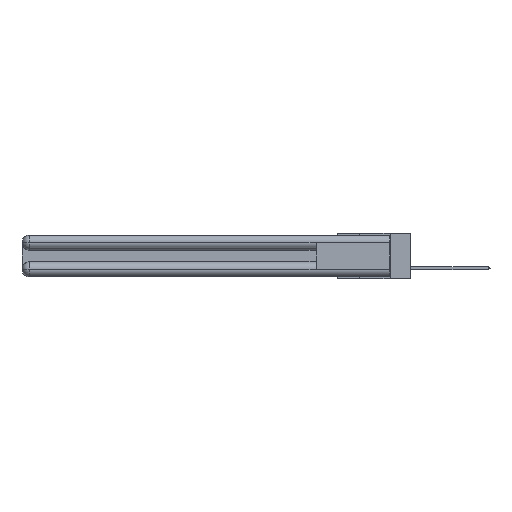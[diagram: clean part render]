
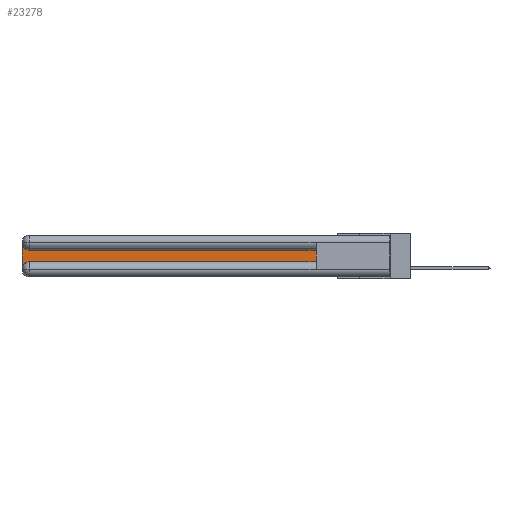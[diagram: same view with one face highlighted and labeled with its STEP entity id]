
A CAD part, left-side view. The second image highlights one B-rep face of the part: STEP entity #23278.
In plain terms, the highlighted planar face has unit normal (-1, 0, 0).
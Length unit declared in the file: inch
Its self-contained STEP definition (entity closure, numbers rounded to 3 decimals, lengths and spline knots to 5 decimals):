
#74 = LINE ( 'NONE', #9603, #21332 ) ;
#1125 = AXIS2_PLACEMENT_3D ( 'NONE', #25899, #30742, #28280 ) ;
#1391 = ORIENTED_EDGE ( 'NONE', *, *, #5317, .T. ) ;
#1719 = CARTESIAN_POINT ( 'NONE',  ( 0.075, 3., -0.1225 ) ) ;
#3764 = LINE ( 'NONE', #11598, #10411 ) ;
#4656 = DIRECTION ( 'NONE',  ( 0., 0., 1. ) ) ;
#5056 = VERTEX_POINT ( 'NONE', #9854 ) ;
#5317 = EDGE_CURVE ( 'NONE', #21313, #30535, #5489, .T. ) ;
#5489 = CIRCLE ( 'NONE', #21120, 0.06 ) ;
#6500 = ORIENTED_EDGE ( 'NONE', *, *, #13131, .T. ) ;
#6522 = CARTESIAN_POINT ( 'NONE',  ( 0.075, 3., -0.2775 ) ) ;
#6923 = PLANE ( 'NONE',  #25638 ) ;
#7786 = EDGE_CURVE ( 'NONE', #10081, #21313, #14411, .T. ) ;
#8075 = VECTOR ( 'NONE', #13045, 39.37008 ) ;
#9087 = DIRECTION ( 'NONE',  ( 1., 0., 0. ) ) ;
#9168 = EDGE_CURVE ( 'NONE', #28397, #5056, #3764, .T. ) ;
#9603 = CARTESIAN_POINT ( 'NONE',  ( 0.075, 0.6, -0.1225 ) ) ;
#9854 = CARTESIAN_POINT ( 'NONE',  ( 0.075, 0.6, -0.1225 ) ) ;
#10081 = VERTEX_POINT ( 'NONE', #17074 ) ;
#10411 = VECTOR ( 'NONE', #4656, 39.37008 ) ;
#10734 = EDGE_LOOP ( 'NONE', ( #6500, #12149, #11460, #1391, #21352, #25869 ) ) ;
#11460 = ORIENTED_EDGE ( 'NONE', *, *, #7786, .T. ) ;
#11598 = CARTESIAN_POINT ( 'NONE',  ( 0.075, 0.6, -0.2175 ) ) ;
#11675 = DIRECTION ( 'NONE',  ( 0., 1., 0. ) ) ;
#12127 = LINE ( 'NONE', #16819, #27448 ) ;
#12149 = ORIENTED_EDGE ( 'NONE', *, *, #28675, .T. ) ;
#13045 = DIRECTION ( 'NONE',  ( 0., 0., -1. ) ) ;
#13131 = EDGE_CURVE ( 'NONE', #5056, #13532, #74, .T. ) ;
#13532 = VERTEX_POINT ( 'NONE', #26546 ) ;
#14411 = LINE ( 'NONE', #17759, #8075 ) ;
#15906 = CARTESIAN_POINT ( 'NONE',  ( 0.075, 2.94, -0.2775 ) ) ;
#16819 = CARTESIAN_POINT ( 'NONE',  ( 0.075, 0.6, -0.2175 ) ) ;
#17074 = CARTESIAN_POINT ( 'NONE',  ( 0.075, 3., -0.0625 ) ) ;
#17759 = CARTESIAN_POINT ( 'NONE',  ( 0.075, 3., -0.2175 ) ) ;
#19348 = CIRCLE ( 'NONE', #1125, 0.06 ) ;
#19451 = DIRECTION ( 'NONE',  ( 0., -1., 0. ) ) ;
#20620 = DIRECTION ( 'NONE',  ( 0., 0., -1. ) ) ;
#21012 = EDGE_CURVE ( 'NONE', #30535, #28397, #12127, .T. ) ;
#21120 = AXIS2_PLACEMENT_3D ( 'NONE', #15906, #25330, #20620 ) ;
#21313 = VERTEX_POINT ( 'NONE', #6522 ) ;
#21332 = VECTOR ( 'NONE', #11675, 39.37008 ) ;
#21352 = ORIENTED_EDGE ( 'NONE', *, *, #21012, .T. ) ;
#22069 = FACE_OUTER_BOUND ( 'NONE', #10734, .T. ) ;
#23169 = DIRECTION ( 'NONE',  ( 0., 0., -1. ) ) ;
#23278 = ADVANCED_FACE ( 'NONE', ( #22069 ), #6923, .F. ) ;
#23506 = CARTESIAN_POINT ( 'NONE',  ( 0.075, 2.94, -0.2175 ) ) ;
#24138 = CARTESIAN_POINT ( 'NONE',  ( 0.075, 0.6, -0.2175 ) ) ;
#25330 = DIRECTION ( 'NONE',  ( 1., 0., 0. ) ) ;
#25638 = AXIS2_PLACEMENT_3D ( 'NONE', #1719, #9087, #23169 ) ;
#25869 = ORIENTED_EDGE ( 'NONE', *, *, #9168, .T. ) ;
#25899 = CARTESIAN_POINT ( 'NONE',  ( 0.075, 2.94, -0.0625 ) ) ;
#26546 = CARTESIAN_POINT ( 'NONE',  ( 0.075, 2.94, -0.1225 ) ) ;
#27448 = VECTOR ( 'NONE', #19451, 39.37008 ) ;
#28280 = DIRECTION ( 'NONE',  ( 0., 0., -1. ) ) ;
#28397 = VERTEX_POINT ( 'NONE', #24138 ) ;
#28675 = EDGE_CURVE ( 'NONE', #13532, #10081, #19348, .T. ) ;
#30535 = VERTEX_POINT ( 'NONE', #23506 ) ;
#30742 = DIRECTION ( 'NONE',  ( 1., 0., 0. ) ) ;
